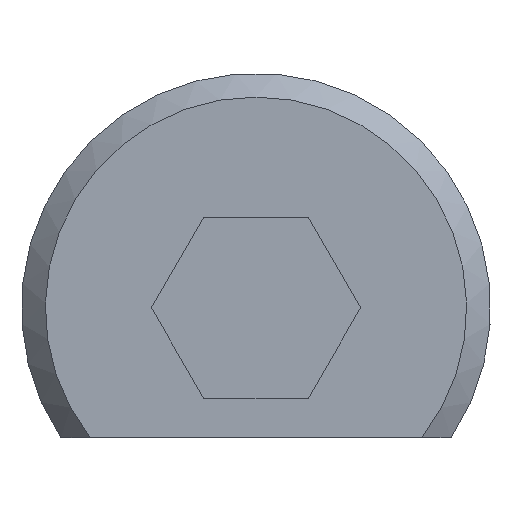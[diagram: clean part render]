
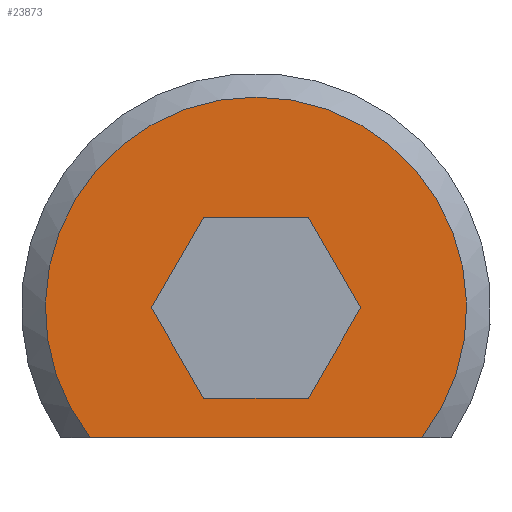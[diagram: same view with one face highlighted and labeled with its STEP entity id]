
A CAD part, left-side view. The second image highlights one B-rep face of the part: STEP entity #23873.
In plain terms, the highlighted planar face has unit normal (-1, 0, 0).
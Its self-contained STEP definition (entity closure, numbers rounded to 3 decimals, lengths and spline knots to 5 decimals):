
#223 = CARTESIAN_POINT ( 'NONE',  ( -0.25, 0.16445, 0. ) ) ;
#319 = ORIENTED_EDGE ( 'NONE', *, *, #25793, .F. ) ;
#1984 = DIRECTION ( 'NONE',  ( 0., 0.5, -0.866 ) ) ;
#2620 = LINE ( 'NONE', #7745, #17522 ) ;
#3189 = CARTESIAN_POINT ( 'NONE',  ( -0.25, 0.08223, -0.14242 ) ) ;
#4061 = FACE_OUTER_BOUND ( 'NONE', #27530, .T. ) ;
#4539 = DIRECTION ( 'NONE',  ( 0., 0.5, 0.866 ) ) ;
#4618 = CARTESIAN_POINT ( 'NONE',  ( -0.25, -0.08223, -0.14242 ) ) ;
#4719 = VERTEX_POINT ( 'NONE', #4618 ) ;
#4832 = EDGE_CURVE ( 'NONE', #21522, #36205, #2620, .T. ) ;
#5958 = ORIENTED_EDGE ( 'NONE', *, *, #4832, .F. ) ;
#7116 = DIRECTION ( 'NONE',  ( -1., 0., 0. ) ) ;
#7242 = VERTEX_POINT ( 'NONE', #27481 ) ;
#7249 = EDGE_CURVE ( 'NONE', #7242, #30852, #13217, .T. ) ;
#7745 = CARTESIAN_POINT ( 'NONE',  ( -0.25, 0.08223, 0.14242 ) ) ;
#9429 = CARTESIAN_POINT ( 'NONE',  ( -0.25, 0.16445, 0. ) ) ;
#10063 = LINE ( 'NONE', #20464, #32256 ) ;
#10375 = FACE_BOUND ( 'NONE', #17893, .T. ) ;
#11317 = DIRECTION ( 'NONE',  ( 0., -0.5, 0.866 ) ) ;
#11813 = ORIENTED_EDGE ( 'NONE', *, *, #17941, .F. ) ;
#13098 = CARTESIAN_POINT ( 'NONE',  ( -0.25, -0.08223, 0.14242 ) ) ;
#13111 = ORIENTED_EDGE ( 'NONE', *, *, #29066, .T. ) ;
#13217 = CIRCLE ( 'NONE', #17044, 0.33125 ) ;
#13525 = CARTESIAN_POINT ( 'NONE',  ( -0.25, -0.16445, 0. ) ) ;
#13727 = DIRECTION ( 'NONE',  ( -1., 0., 0. ) ) ;
#14433 = LINE ( 'NONE', #223, #28895 ) ;
#14738 = CARTESIAN_POINT ( 'NONE',  ( -0.25, -0.16445, 0. ) ) ;
#14982 = VERTEX_POINT ( 'NONE', #3189 ) ;
#15160 = LINE ( 'NONE', #31791, #26437 ) ;
#16261 = VERTEX_POINT ( 'NONE', #13098 ) ;
#17044 = AXIS2_PLACEMENT_3D ( 'NONE', #34221, #13727, #19891 ) ;
#17261 = DIRECTION ( 'NONE',  ( 0., -0.5, -0.866 ) ) ;
#17522 = VECTOR ( 'NONE', #1984, 39.37008 ) ;
#17893 = EDGE_LOOP ( 'NONE', ( #33377, #319, #5958, #27015, #11813, #18610 ) ) ;
#17941 = EDGE_CURVE ( 'NONE', #26323, #16261, #28971, .T. ) ;
#18610 = ORIENTED_EDGE ( 'NONE', *, *, #30790, .F. ) ;
#18633 = CARTESIAN_POINT ( 'NONE',  ( -0.25, 0., 0. ) ) ;
#19891 = DIRECTION ( 'NONE',  ( 0., 0., 1. ) ) ;
#20464 = CARTESIAN_POINT ( 'NONE',  ( -0.25, 0.08223, -0.14242 ) ) ;
#21216 = LINE ( 'NONE', #29257, #23012 ) ;
#21522 = VERTEX_POINT ( 'NONE', #23195 ) ;
#21528 = DIRECTION ( 'NONE',  ( 0., -1., 0. ) ) ;
#23012 = VECTOR ( 'NONE', #23811, 39.37008 ) ;
#23195 = CARTESIAN_POINT ( 'NONE',  ( -0.25, 0.08223, 0.14242 ) ) ;
#23811 = DIRECTION ( 'NONE',  ( 0., 1., 0. ) ) ;
#23873 = ADVANCED_FACE ( 'NONE', ( #4061, #10375 ), #27467, .T. ) ;
#23994 = VECTOR ( 'NONE', #4539, 39.37008 ) ;
#25793 = EDGE_CURVE ( 'NONE', #36205, #14982, #14433, .T. ) ;
#26079 = CARTESIAN_POINT ( 'NONE',  ( -0.25, 0.26053, -0.20458 ) ) ;
#26166 = VECTOR ( 'NONE', #21528, 39.37008 ) ;
#26323 = VERTEX_POINT ( 'NONE', #14738 ) ;
#26391 = EDGE_CURVE ( 'NONE', #16261, #21522, #21216, .T. ) ;
#26437 = VECTOR ( 'NONE', #11317, 39.37008 ) ;
#27015 = ORIENTED_EDGE ( 'NONE', *, *, #26391, .F. ) ;
#27087 = DIRECTION ( 'NONE',  ( 0., 0., 1. ) ) ;
#27467 = PLANE ( 'NONE',  #29802 ) ;
#27481 = CARTESIAN_POINT ( 'NONE',  ( -0.25, -0.26053, -0.20458 ) ) ;
#27530 = EDGE_LOOP ( 'NONE', ( #13111, #31187 ) ) ;
#28459 = LINE ( 'NONE', #35967, #26166 ) ;
#28460 = EDGE_CURVE ( 'NONE', #14982, #4719, #10063, .T. ) ;
#28895 = VECTOR ( 'NONE', #17261, 39.37008 ) ;
#28971 = LINE ( 'NONE', #13525, #23994 ) ;
#29066 = EDGE_CURVE ( 'NONE', #30852, #7242, #28459, .T. ) ;
#29257 = CARTESIAN_POINT ( 'NONE',  ( -0.25, -0.08223, 0.14242 ) ) ;
#29423 = DIRECTION ( 'NONE',  ( 0., -1., 0. ) ) ;
#29802 = AXIS2_PLACEMENT_3D ( 'NONE', #18633, #7116, #27087 ) ;
#30790 = EDGE_CURVE ( 'NONE', #4719, #26323, #15160, .T. ) ;
#30852 = VERTEX_POINT ( 'NONE', #26079 ) ;
#31187 = ORIENTED_EDGE ( 'NONE', *, *, #7249, .T. ) ;
#31791 = CARTESIAN_POINT ( 'NONE',  ( -0.25, -0.08223, -0.14242 ) ) ;
#32256 = VECTOR ( 'NONE', #29423, 39.37008 ) ;
#33377 = ORIENTED_EDGE ( 'NONE', *, *, #28460, .F. ) ;
#34221 = CARTESIAN_POINT ( 'NONE',  ( -0.25, 0., 0. ) ) ;
#35967 = CARTESIAN_POINT ( 'NONE',  ( -0.25, 0.3068, -0.20458 ) ) ;
#36205 = VERTEX_POINT ( 'NONE', #9429 ) ;
